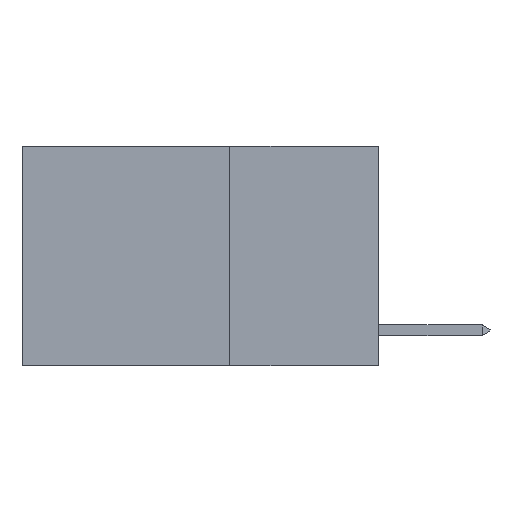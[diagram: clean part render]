
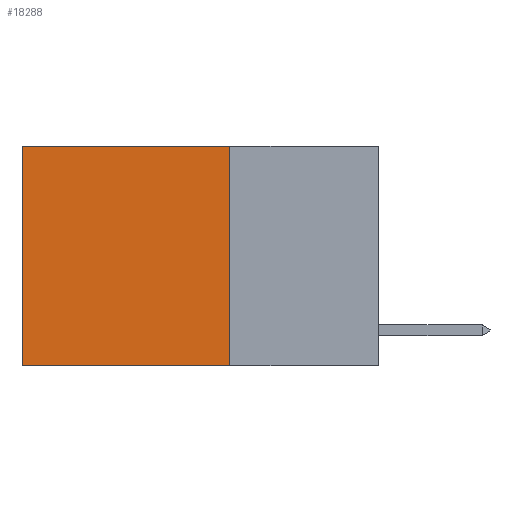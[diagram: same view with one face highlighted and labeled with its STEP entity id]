
A CAD part, left-side view. The second image highlights one B-rep face of the part: STEP entity #18288.
In plain terms, the highlighted planar face has unit normal (-1, 0, 0).
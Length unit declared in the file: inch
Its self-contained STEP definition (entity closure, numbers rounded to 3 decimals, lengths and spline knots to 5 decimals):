
#18 = ORIENTED_EDGE ( 'NONE', *, *, #1127, .T. ) ;
#1127 = EDGE_CURVE ( 'NONE', #19375, #18198, #21380, .T. ) ;
#1172 = EDGE_LOOP ( 'NONE', ( #18, #7320, #18887, #4801 ) ) ;
#3299 = CARTESIAN_POINT ( 'NONE',  ( 0.2625, 0.25, 0. ) ) ;
#4052 = VECTOR ( 'NONE', #8314, 39.37008 ) ;
#4078 = VERTEX_POINT ( 'NONE', #23280 ) ;
#4527 = EDGE_CURVE ( 'NONE', #18093, #19375, #9447, .T. ) ;
#4801 = ORIENTED_EDGE ( 'NONE', *, *, #4527, .T. ) ;
#6335 = CARTESIAN_POINT ( 'NONE',  ( 0.2625, 0.25, 0. ) ) ;
#7320 = ORIENTED_EDGE ( 'NONE', *, *, #10470, .F. ) ;
#7492 = FACE_OUTER_BOUND ( 'NONE', #1172, .T. ) ;
#8314 = DIRECTION ( 'NONE',  ( 0., 0., -1. ) ) ;
#9222 = CARTESIAN_POINT ( 'NONE',  ( 0.2625, 0.6, 0. ) ) ;
#9447 = LINE ( 'NONE', #24616, #19071 ) ;
#9789 = PLANE ( 'NONE',  #21960 ) ;
#10430 = DIRECTION ( 'NONE',  ( 0., 0., -1. ) ) ;
#10470 = EDGE_CURVE ( 'NONE', #4078, #18198, #16978, .T. ) ;
#10592 = DIRECTION ( 'NONE',  ( 0., 1., 0. ) ) ;
#11103 = VECTOR ( 'NONE', #17448, 39.37008 ) ;
#11698 = DIRECTION ( 'NONE',  ( 1., 0., 0. ) ) ;
#12474 = VECTOR ( 'NONE', #10592, 39.37008 ) ;
#14374 = LINE ( 'NONE', #6335, #4052 ) ;
#16978 = LINE ( 'NONE', #22175, #12474 ) ;
#17414 = CARTESIAN_POINT ( 'NONE',  ( 0.2625, 0.25, 0. ) ) ;
#17448 = DIRECTION ( 'NONE',  ( 0., 0., -1. ) ) ;
#18052 = CARTESIAN_POINT ( 'NONE',  ( 0.2625, 0.6, 0. ) ) ;
#18093 = VERTEX_POINT ( 'NONE', #3299 ) ;
#18198 = VERTEX_POINT ( 'NONE', #25008 ) ;
#18288 = ADVANCED_FACE ( 'NONE', ( #7492 ), #9789, .F. ) ;
#18887 = ORIENTED_EDGE ( 'NONE', *, *, #19535, .F. ) ;
#19071 = VECTOR ( 'NONE', #22736, 39.37008 ) ;
#19375 = VERTEX_POINT ( 'NONE', #9222 ) ;
#19535 = EDGE_CURVE ( 'NONE', #18093, #4078, #14374, .T. ) ;
#21380 = LINE ( 'NONE', #18052, #11103 ) ;
#21960 = AXIS2_PLACEMENT_3D ( 'NONE', #17414, #11698, #10430 ) ;
#22175 = CARTESIAN_POINT ( 'NONE',  ( 0.2625, 0.25, -0.37 ) ) ;
#22736 = DIRECTION ( 'NONE',  ( 0., 1., 0. ) ) ;
#23280 = CARTESIAN_POINT ( 'NONE',  ( 0.2625, 0.25, -0.37 ) ) ;
#24616 = CARTESIAN_POINT ( 'NONE',  ( 0.2625, 0.25, 0. ) ) ;
#25008 = CARTESIAN_POINT ( 'NONE',  ( 0.2625, 0.6, -0.37 ) ) ;
